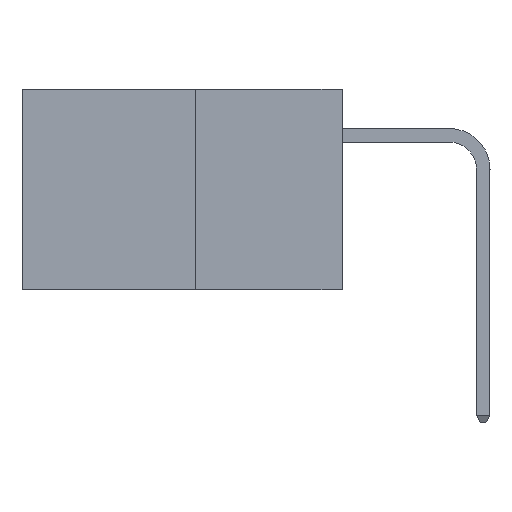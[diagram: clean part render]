
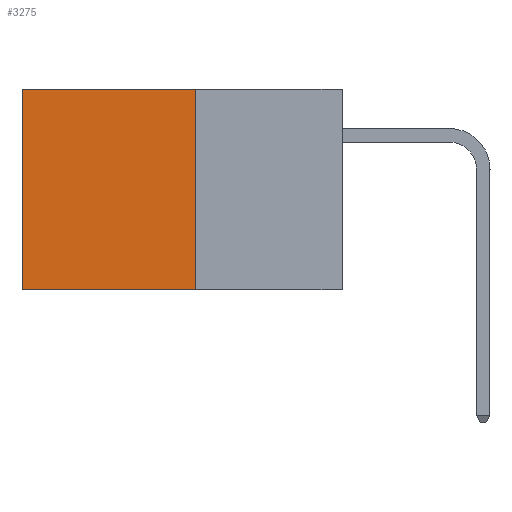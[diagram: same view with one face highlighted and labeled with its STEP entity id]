
A CAD part, left-side view. The second image highlights one B-rep face of the part: STEP entity #3275.
In plain terms, the highlighted planar face has unit normal (-1, 0, 0).
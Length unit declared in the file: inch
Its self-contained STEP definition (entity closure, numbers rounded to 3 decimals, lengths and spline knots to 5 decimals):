
#1223 = VERTEX_POINT ( 'NONE', #5638 ) ;
#1428 = ORIENTED_EDGE ( 'NONE', *, *, #4195, .F. ) ;
#1654 = ORIENTED_EDGE ( 'NONE', *, *, #12093, .T. ) ;
#2380 = DIRECTION ( 'NONE',  ( 0., 1., 0. ) ) ;
#2456 = DIRECTION ( 'NONE',  ( 0., 0., -1. ) ) ;
#2646 = DIRECTION ( 'NONE',  ( 1., 0., 0. ) ) ;
#2690 = VECTOR ( 'NONE', #7692, 39.37008 ) ;
#2804 = CARTESIAN_POINT ( 'NONE',  ( 0.277, 0.59, -0.37 ) ) ;
#2812 = PLANE ( 'NONE',  #9871 ) ;
#2871 = CARTESIAN_POINT ( 'NONE',  ( 0.277, 0.27, -0.37 ) ) ;
#2990 = DIRECTION ( 'NONE',  ( 0., 1., 0. ) ) ;
#3116 = CARTESIAN_POINT ( 'NONE',  ( 0.277, 0.27, 0. ) ) ;
#3275 = ADVANCED_FACE ( 'NONE', ( #11817 ), #2812, .F. ) ;
#3399 = CARTESIAN_POINT ( 'NONE',  ( 0.277, 0.27, 0. ) ) ;
#3522 = VERTEX_POINT ( 'NONE', #10348 ) ;
#3722 = DIRECTION ( 'NONE',  ( 0., 0., -1. ) ) ;
#4164 = VERTEX_POINT ( 'NONE', #3116 ) ;
#4195 = EDGE_CURVE ( 'NONE', #1223, #3522, #9370, .T. ) ;
#5638 = CARTESIAN_POINT ( 'NONE',  ( 0.277, 0.27, -0.37 ) ) ;
#5936 = EDGE_CURVE ( 'NONE', #8750, #3522, #10356, .T. ) ;
#6620 = CARTESIAN_POINT ( 'NONE',  ( 0.277, 0.27, -0.37 ) ) ;
#6867 = VECTOR ( 'NONE', #2990, 39.37008 ) ;
#7328 = ORIENTED_EDGE ( 'NONE', *, *, #9455, .F. ) ;
#7692 = DIRECTION ( 'NONE',  ( 0., 0., -1. ) ) ;
#7786 = ORIENTED_EDGE ( 'NONE', *, *, #5936, .T. ) ;
#8013 = LINE ( 'NONE', #3399, #12268 ) ;
#8750 = VERTEX_POINT ( 'NONE', #11712 ) ;
#9370 = LINE ( 'NONE', #2871, #6867 ) ;
#9455 = EDGE_CURVE ( 'NONE', #4164, #1223, #9903, .T. ) ;
#9787 = EDGE_LOOP ( 'NONE', ( #7786, #1428, #7328, #1654 ) ) ;
#9871 = AXIS2_PLACEMENT_3D ( 'NONE', #11148, #2646, #2456 ) ;
#9903 = LINE ( 'NONE', #6620, #12289 ) ;
#10348 = CARTESIAN_POINT ( 'NONE',  ( 0.277, 0.59, -0.37 ) ) ;
#10356 = LINE ( 'NONE', #2804, #2690 ) ;
#11148 = CARTESIAN_POINT ( 'NONE',  ( 0.277, 0.27, -0.37 ) ) ;
#11712 = CARTESIAN_POINT ( 'NONE',  ( 0.277, 0.59, 0. ) ) ;
#11817 = FACE_OUTER_BOUND ( 'NONE', #9787, .T. ) ;
#12093 = EDGE_CURVE ( 'NONE', #4164, #8750, #8013, .T. ) ;
#12268 = VECTOR ( 'NONE', #2380, 39.37008 ) ;
#12289 = VECTOR ( 'NONE', #3722, 39.37008 ) ;
